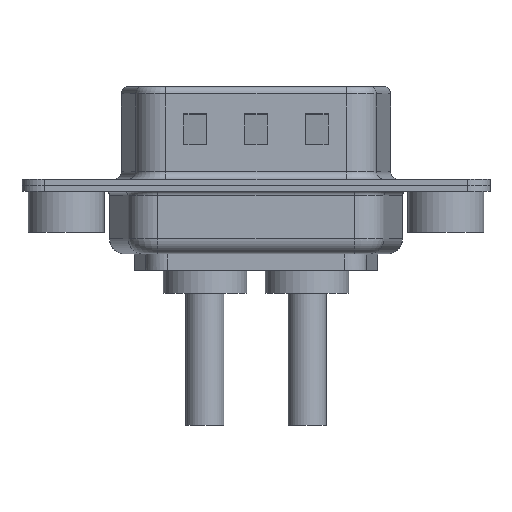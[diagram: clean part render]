
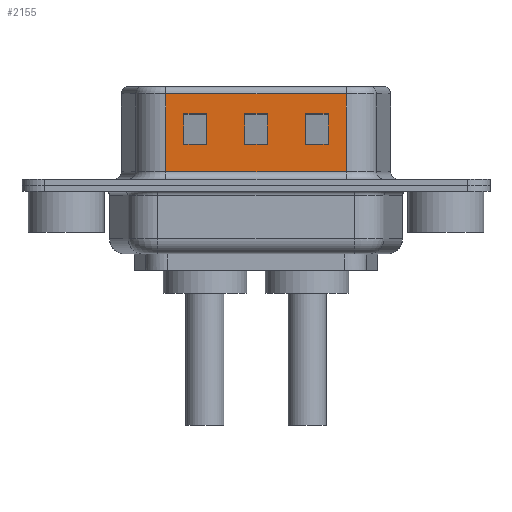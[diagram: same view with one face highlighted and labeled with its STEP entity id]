
A CAD part, front view. The second image highlights one B-rep face of the part: STEP entity #2155.
In plain terms, the highlighted planar face has unit normal (0, -1, 0).
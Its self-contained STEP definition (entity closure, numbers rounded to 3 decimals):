
#154 = EDGE_LOOP ( 'NONE', ( #8314, #2184, #6650, #16178 ) ) ;
#271 = DIRECTION ( 'NONE',  ( 0., 0., 1. ) ) ;
#366 = VECTOR ( 'NONE', #10612, 1000. ) ;
#368 = DIRECTION ( 'NONE',  ( 1., 0., 0. ) ) ;
#402 = LINE ( 'NONE', #6997, #10191 ) ;
#437 = LINE ( 'NONE', #4150, #14205 ) ;
#473 = FACE_BOUND ( 'NONE', #5150, .T. ) ;
#711 = EDGE_CURVE ( 'NONE', #1802, #6274, #17362, .T. ) ;
#734 = ORIENTED_EDGE ( 'NONE', *, *, #13553, .T. ) ;
#843 = VERTEX_POINT ( 'NONE', #9070 ) ;
#1011 = EDGE_CURVE ( 'NONE', #1802, #8104, #14761, .T. ) ;
#1167 = LINE ( 'NONE', #5916, #11807 ) ;
#1324 = VECTOR ( 'NONE', #4860, 1000. ) ;
#1445 = ORIENTED_EDGE ( 'NONE', *, *, #15383, .T. ) ;
#1516 = CARTESIAN_POINT ( 'NONE',  ( 17.25, -4.58, 2.705 ) ) ;
#1534 = ORIENTED_EDGE ( 'NONE', *, *, #10515, .T. ) ;
#1563 = LINE ( 'NONE', #11820, #8245 ) ;
#1730 = LINE ( 'NONE', #7062, #4853 ) ;
#1802 = VERTEX_POINT ( 'NONE', #9970 ) ;
#2155 = ADVANCED_FACE ( 'NONE', ( #473, #7137, #3966, #10667 ), #9201, .F. ) ;
#2184 = ORIENTED_EDGE ( 'NONE', *, *, #1011, .T. ) ;
#2379 = LINE ( 'NONE', #5793, #2790 ) ;
#2453 = CARTESIAN_POINT ( 'NONE',  ( 7.75, -4.58, 2.705 ) ) ;
#2456 = LINE ( 'NONE', #12926, #17201 ) ;
#2751 = EDGE_CURVE ( 'NONE', #8104, #7820, #11918, .T. ) ;
#2790 = VECTOR ( 'NONE', #15191, 1000. ) ;
#2993 = CARTESIAN_POINT ( 'NONE',  ( 6.55, -4.58, 0.9 ) ) ;
#3080 = VECTOR ( 'NONE', #12085, 1000. ) ;
#3269 = VECTOR ( 'NONE', #16330, 1000. ) ;
#3483 = VECTOR ( 'NONE', #7684, 1000. ) ;
#3624 = CARTESIAN_POINT ( 'NONE',  ( 9.25, -4.58, 2.705 ) ) ;
#3966 = FACE_BOUND ( 'NONE', #16446, .T. ) ;
#4031 = CARTESIAN_POINT ( 'NONE',  ( 18.45, -4.58, 6.02 ) ) ;
#4070 = LINE ( 'NONE', #15864, #14773 ) ;
#4150 = CARTESIAN_POINT ( 'NONE',  ( 22.45, -4.58, 2.705 ) ) ;
#4298 = CARTESIAN_POINT ( 'NONE',  ( 11.75, -4.58, 4.705 ) ) ;
#4572 = EDGE_CURVE ( 'NONE', #843, #15123, #2456, .T. ) ;
#4767 = EDGE_CURVE ( 'NONE', #8824, #16157, #14180, .T. ) ;
#4795 = VECTOR ( 'NONE', #6251, 1000. ) ;
#4852 = LINE ( 'NONE', #8839, #1324 ) ;
#4853 = VECTOR ( 'NONE', #368, 1000. ) ;
#4860 = DIRECTION ( 'NONE',  ( 1., 0., 0. ) ) ;
#4995 = CARTESIAN_POINT ( 'NONE',  ( 6.55, -4.58, 6.02 ) ) ;
#5043 = EDGE_CURVE ( 'NONE', #15123, #6977, #13970, .T. ) ;
#5083 = CARTESIAN_POINT ( 'NONE',  ( 9.25, -4.58, 4.705 ) ) ;
#5150 = EDGE_LOOP ( 'NONE', ( #10550, #11448, #11255, #14606 ) ) ;
#5793 = CARTESIAN_POINT ( 'NONE',  ( 14.45, -4.58, 4.705 ) ) ;
#5916 = CARTESIAN_POINT ( 'NONE',  ( 7.75, -4.58, 6.52 ) ) ;
#6053 = EDGE_CURVE ( 'NONE', #6868, #843, #10206, .T. ) ;
#6251 = DIRECTION ( 'NONE',  ( 0., 0., -1. ) ) ;
#6274 = VERTEX_POINT ( 'NONE', #12071 ) ;
#6431 = VERTEX_POINT ( 'NONE', #9032 ) ;
#6570 = VERTEX_POINT ( 'NONE', #7952 ) ;
#6650 = ORIENTED_EDGE ( 'NONE', *, *, #2751, .T. ) ;
#6682 = EDGE_CURVE ( 'NONE', #16157, #14963, #402, .T. ) ;
#6868 = VERTEX_POINT ( 'NONE', #7057 ) ;
#6977 = VERTEX_POINT ( 'NONE', #13699 ) ;
#6993 = CARTESIAN_POINT ( 'NONE',  ( 9.25, -4.58, 6.52 ) ) ;
#6997 = CARTESIAN_POINT ( 'NONE',  ( 14.45, -4.58, 2.705 ) ) ;
#7057 = CARTESIAN_POINT ( 'NONE',  ( 13.25, -4.58, 2.705 ) ) ;
#7062 = CARTESIAN_POINT ( 'NONE',  ( 18.45, -4.58, 0.9 ) ) ;
#7137 = FACE_BOUND ( 'NONE', #14458, .T. ) ;
#7424 = CARTESIAN_POINT ( 'NONE',  ( 6.55, -4.58, 6.52 ) ) ;
#7684 = DIRECTION ( 'NONE',  ( 0., 0., -1. ) ) ;
#7820 = VERTEX_POINT ( 'NONE', #2993 ) ;
#7952 = CARTESIAN_POINT ( 'NONE',  ( 7.75, -4.58, 4.705 ) ) ;
#7959 = ORIENTED_EDGE ( 'NONE', *, *, #12870, .T. ) ;
#8024 = VERTEX_POINT ( 'NONE', #15646 ) ;
#8104 = VERTEX_POINT ( 'NONE', #4995 ) ;
#8216 = CARTESIAN_POINT ( 'NONE',  ( 15.75, -4.58, 6.52 ) ) ;
#8245 = VECTOR ( 'NONE', #13160, 1000. ) ;
#8256 = DIRECTION ( 'NONE',  ( -1., 0., 0. ) ) ;
#8314 = ORIENTED_EDGE ( 'NONE', *, *, #711, .F. ) ;
#8354 = VECTOR ( 'NONE', #271, 1000. ) ;
#8685 = EDGE_CURVE ( 'NONE', #14963, #6570, #1167, .T. ) ;
#8824 = VERTEX_POINT ( 'NONE', #5083 ) ;
#8839 = CARTESIAN_POINT ( 'NONE',  ( 22.45, -4.58, 4.705 ) ) ;
#9032 = CARTESIAN_POINT ( 'NONE',  ( 15.75, -4.58, 4.705 ) ) ;
#9068 = DIRECTION ( 'NONE',  ( 0., 0., 1. ) ) ;
#9070 = CARTESIAN_POINT ( 'NONE',  ( 11.75, -4.58, 2.705 ) ) ;
#9201 = PLANE ( 'NONE',  #17164 ) ;
#9602 = CARTESIAN_POINT ( 'NONE',  ( 18.45, -4.58, 6.52 ) ) ;
#9970 = CARTESIAN_POINT ( 'NONE',  ( 18.45, -4.58, 6.02 ) ) ;
#10191 = VECTOR ( 'NONE', #12100, 1000. ) ;
#10206 = LINE ( 'NONE', #14787, #3080 ) ;
#10301 = EDGE_CURVE ( 'NONE', #7820, #6274, #1730, .T. ) ;
#10515 = EDGE_CURVE ( 'NONE', #6431, #13983, #4852, .T. ) ;
#10550 = ORIENTED_EDGE ( 'NONE', *, *, #4767, .T. ) ;
#10554 = CARTESIAN_POINT ( 'NONE',  ( 18.45, -4.58, 6.52 ) ) ;
#10612 = DIRECTION ( 'NONE',  ( 0., 0., -1. ) ) ;
#10667 = FACE_OUTER_BOUND ( 'NONE', #154, .T. ) ;
#11177 = VECTOR ( 'NONE', #12112, 1000. ) ;
#11255 = ORIENTED_EDGE ( 'NONE', *, *, #8685, .T. ) ;
#11448 = ORIENTED_EDGE ( 'NONE', *, *, #6682, .T. ) ;
#11577 = ORIENTED_EDGE ( 'NONE', *, *, #5043, .T. ) ;
#11807 = VECTOR ( 'NONE', #13954, 1000. ) ;
#11820 = CARTESIAN_POINT ( 'NONE',  ( 13.25, -4.58, 6.52 ) ) ;
#11833 = DIRECTION ( 'NONE',  ( 0., 1., 0. ) ) ;
#11913 = LINE ( 'NONE', #8216, #8354 ) ;
#11918 = LINE ( 'NONE', #7424, #4795 ) ;
#12071 = CARTESIAN_POINT ( 'NONE',  ( 18.45, -4.58, 0.9 ) ) ;
#12085 = DIRECTION ( 'NONE',  ( -1., 0., 0. ) ) ;
#12100 = DIRECTION ( 'NONE',  ( -1., 0., 0. ) ) ;
#12112 = DIRECTION ( 'NONE',  ( -1., 0., 0. ) ) ;
#12804 = ORIENTED_EDGE ( 'NONE', *, *, #16226, .T. ) ;
#12870 = EDGE_CURVE ( 'NONE', #8024, #6431, #11913, .T. ) ;
#12926 = CARTESIAN_POINT ( 'NONE',  ( 11.75, -4.58, 6.52 ) ) ;
#13160 = DIRECTION ( 'NONE',  ( 0., 0., -1. ) ) ;
#13553 = EDGE_CURVE ( 'NONE', #14128, #8024, #437, .T. ) ;
#13699 = CARTESIAN_POINT ( 'NONE',  ( 13.25, -4.58, 4.705 ) ) ;
#13954 = DIRECTION ( 'NONE',  ( 0., 0., 1. ) ) ;
#13961 = ORIENTED_EDGE ( 'NONE', *, *, #4572, .T. ) ;
#13970 = LINE ( 'NONE', #14249, #3269 ) ;
#13983 = VERTEX_POINT ( 'NONE', #15788 ) ;
#14128 = VERTEX_POINT ( 'NONE', #1516 ) ;
#14180 = LINE ( 'NONE', #6993, #3483 ) ;
#14205 = VECTOR ( 'NONE', #8256, 1000. ) ;
#14249 = CARTESIAN_POINT ( 'NONE',  ( 18.45, -4.58, 4.705 ) ) ;
#14458 = EDGE_LOOP ( 'NONE', ( #1445, #734, #7959, #1534 ) ) ;
#14606 = ORIENTED_EDGE ( 'NONE', *, *, #16733, .T. ) ;
#14761 = LINE ( 'NONE', #4031, #11177 ) ;
#14773 = VECTOR ( 'NONE', #17182, 1000. ) ;
#14787 = CARTESIAN_POINT ( 'NONE',  ( 18.45, -4.58, 2.705 ) ) ;
#14963 = VERTEX_POINT ( 'NONE', #2453 ) ;
#15123 = VERTEX_POINT ( 'NONE', #4298 ) ;
#15191 = DIRECTION ( 'NONE',  ( 1., 0., 0. ) ) ;
#15383 = EDGE_CURVE ( 'NONE', #13983, #14128, #4070, .T. ) ;
#15646 = CARTESIAN_POINT ( 'NONE',  ( 15.75, -4.58, 2.705 ) ) ;
#15788 = CARTESIAN_POINT ( 'NONE',  ( 17.25, -4.58, 4.705 ) ) ;
#15864 = CARTESIAN_POINT ( 'NONE',  ( 17.25, -4.58, 6.52 ) ) ;
#16157 = VERTEX_POINT ( 'NONE', #3624 ) ;
#16178 = ORIENTED_EDGE ( 'NONE', *, *, #10301, .T. ) ;
#16226 = EDGE_CURVE ( 'NONE', #6977, #6868, #1563, .T. ) ;
#16301 = ORIENTED_EDGE ( 'NONE', *, *, #6053, .T. ) ;
#16330 = DIRECTION ( 'NONE',  ( 1., 0., 0. ) ) ;
#16446 = EDGE_LOOP ( 'NONE', ( #11577, #12804, #16301, #13961 ) ) ;
#16700 = DIRECTION ( 'NONE',  ( 0., 0., 1. ) ) ;
#16733 = EDGE_CURVE ( 'NONE', #6570, #8824, #2379, .T. ) ;
#17164 = AXIS2_PLACEMENT_3D ( 'NONE', #9602, #11833, #9068 ) ;
#17182 = DIRECTION ( 'NONE',  ( 0., 0., -1. ) ) ;
#17201 = VECTOR ( 'NONE', #16700, 1000. ) ;
#17362 = LINE ( 'NONE', #10554, #366 ) ;
